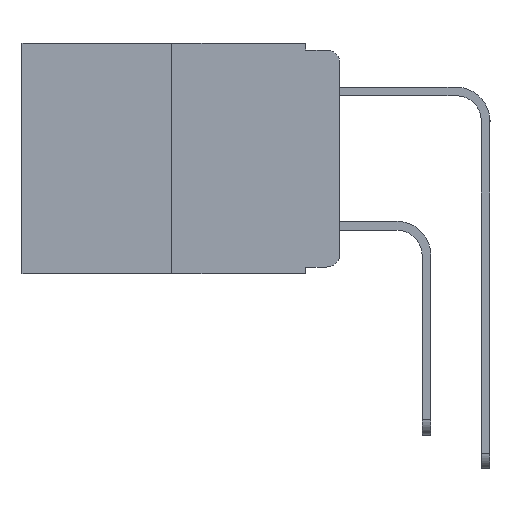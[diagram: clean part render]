
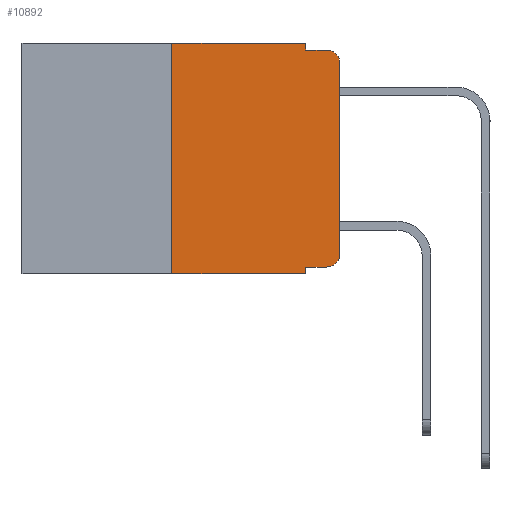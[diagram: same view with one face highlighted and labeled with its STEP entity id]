
A CAD part, left-side view. The second image highlights one B-rep face of the part: STEP entity #10892.
In plain terms, the highlighted planar face has unit normal (-1, 0, 0).
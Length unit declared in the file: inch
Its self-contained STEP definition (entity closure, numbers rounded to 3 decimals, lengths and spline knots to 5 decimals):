
#86 = VERTEX_POINT ( 'NONE', #1285 ) ;
#115 = CARTESIAN_POINT ( 'NONE',  ( 0., 0.051, -0.333 ) ) ;
#425 = VECTOR ( 'NONE', #3945, 39.37008 ) ;
#509 = VERTEX_POINT ( 'NONE', #13855 ) ;
#835 = CARTESIAN_POINT ( 'NONE',  ( 0., 0.02, -0.03 ) ) ;
#933 = LINE ( 'NONE', #15939, #8012 ) ;
#1285 = CARTESIAN_POINT ( 'NONE',  ( 0., 0.051, 0. ) ) ;
#1426 = VECTOR ( 'NONE', #2338, 39.37008 ) ;
#1512 = VERTEX_POINT ( 'NONE', #11597 ) ;
#2338 = DIRECTION ( 'NONE',  ( 0., 0., 1. ) ) ;
#2405 = DIRECTION ( 'NONE',  ( 0., 0., -1. ) ) ;
#2506 = PLANE ( 'NONE',  #4521 ) ;
#2543 = DIRECTION ( 'NONE',  ( -1., 0., 0. ) ) ;
#2708 = CARTESIAN_POINT ( 'NONE',  ( 0., 0., -0.03 ) ) ;
#2984 = AXIS2_PLACEMENT_3D ( 'NONE', #835, #10564, #2405 ) ;
#3136 = VERTEX_POINT ( 'NONE', #115 ) ;
#3711 = VERTEX_POINT ( 'NONE', #16877 ) ;
#3806 = ORIENTED_EDGE ( 'NONE', *, *, #12491, .F. ) ;
#3874 = DIRECTION ( 'NONE',  ( 0., 0., -1. ) ) ;
#3945 = DIRECTION ( 'NONE',  ( 0., -1., 0. ) ) ;
#4009 = CIRCLE ( 'NONE', #4880, 0.02 ) ;
#4450 = LINE ( 'NONE', #14625, #425 ) ;
#4521 = AXIS2_PLACEMENT_3D ( 'NONE', #15959, #8034, #17279 ) ;
#4576 = ORIENTED_EDGE ( 'NONE', *, *, #12466, .T. ) ;
#4861 = LINE ( 'NONE', #15879, #15530 ) ;
#4880 = AXIS2_PLACEMENT_3D ( 'NONE', #10687, #2543, #12038 ) ;
#5078 = ORIENTED_EDGE ( 'NONE', *, *, #12472, .F. ) ;
#5169 = DIRECTION ( 'NONE',  ( 0., -1., 0. ) ) ;
#6206 = ORIENTED_EDGE ( 'NONE', *, *, #12239, .T. ) ;
#6350 = ORIENTED_EDGE ( 'NONE', *, *, #12498, .T. ) ;
#6614 = DIRECTION ( 'NONE',  ( 0., -1., 0. ) ) ;
#6674 = DIRECTION ( 'NONE',  ( 0., 0., 1. ) ) ;
#7125 = VERTEX_POINT ( 'NONE', #2708 ) ;
#7220 = CARTESIAN_POINT ( 'NONE',  ( 0., 0.25, 0. ) ) ;
#7296 = ORIENTED_EDGE ( 'NONE', *, *, #12518, .T. ) ;
#7422 = DIRECTION ( 'NONE',  ( 0., -1., 0. ) ) ;
#8012 = VECTOR ( 'NONE', #6674, 39.37008 ) ;
#8034 = DIRECTION ( 'NONE',  ( 1., 0., 0. ) ) ;
#8382 = CIRCLE ( 'NONE', #2984, 0.02 ) ;
#8410 = VERTEX_POINT ( 'NONE', #8828 ) ;
#8828 = CARTESIAN_POINT ( 'NONE',  ( 0., 0.02, -0.333 ) ) ;
#9134 = CARTESIAN_POINT ( 'NONE',  ( 0., 0., 0. ) ) ;
#9140 = LINE ( 'NONE', #13176, #10414 ) ;
#9146 = VERTEX_POINT ( 'NONE', #7220 ) ;
#9201 = CARTESIAN_POINT ( 'NONE',  ( 0., 0.051, 0. ) ) ;
#9471 = ORIENTED_EDGE ( 'NONE', *, *, #12452, .T. ) ;
#10164 = VERTEX_POINT ( 'NONE', #14168 ) ;
#10378 = CARTESIAN_POINT ( 'NONE',  ( 0., 0.02, -0.01 ) ) ;
#10414 = VECTOR ( 'NONE', #5169, 39.37008 ) ;
#10564 = DIRECTION ( 'NONE',  ( -1., 0., 0. ) ) ;
#10623 = DIRECTION ( 'NONE',  ( 0., 0., -1. ) ) ;
#10687 = CARTESIAN_POINT ( 'NONE',  ( 0., 0.02, -0.313 ) ) ;
#10750 = ORIENTED_EDGE ( 'NONE', *, *, #12494, .F. ) ;
#10892 = ADVANCED_FACE ( 'NONE', ( #11276 ), #2506, .F. ) ;
#11276 = FACE_OUTER_BOUND ( 'NONE', #14150, .T. ) ;
#11597 = CARTESIAN_POINT ( 'NONE',  ( 0., 0.051, -0.343 ) ) ;
#11916 = EDGE_CURVE ( 'NONE', #9146, #86, #9140, .T. ) ;
#11980 = LINE ( 'NONE', #9201, #15124 ) ;
#12038 = DIRECTION ( 'NONE',  ( 0., 0., -1. ) ) ;
#12239 = EDGE_CURVE ( 'NONE', #509, #1512, #16920, .T. ) ;
#12418 = LINE ( 'NONE', #9134, #1426 ) ;
#12452 = EDGE_CURVE ( 'NONE', #3711, #7125, #12418, .T. ) ;
#12466 = EDGE_CURVE ( 'NONE', #7125, #17675, #8382, .T. ) ;
#12469 = EDGE_CURVE ( 'NONE', #10164, #17675, #4861, .T. ) ;
#12472 = EDGE_CURVE ( 'NONE', #86, #10164, #11980, .T. ) ;
#12491 = EDGE_CURVE ( 'NONE', #509, #9146, #933, .T. ) ;
#12494 = EDGE_CURVE ( 'NONE', #3136, #1512, #15937, .T. ) ;
#12498 = EDGE_CURVE ( 'NONE', #3136, #8410, #4450, .T. ) ;
#12518 = EDGE_CURVE ( 'NONE', #8410, #3711, #4009, .T. ) ;
#13176 = CARTESIAN_POINT ( 'NONE',  ( 0., 0.473, 0. ) ) ;
#13490 = ORIENTED_EDGE ( 'NONE', *, *, #11916, .F. ) ;
#13855 = CARTESIAN_POINT ( 'NONE',  ( 0., 0.25, -0.343 ) ) ;
#14071 = CARTESIAN_POINT ( 'NONE',  ( 0., 0.473, -0.343 ) ) ;
#14150 = EDGE_LOOP ( 'NONE', ( #9471, #4576, #15252, #5078, #13490, #3806, #6206, #10750, #6350, #7296 ) ) ;
#14168 = CARTESIAN_POINT ( 'NONE',  ( 0., 0.051, -0.01 ) ) ;
#14625 = CARTESIAN_POINT ( 'NONE',  ( 0., 0.051, -0.333 ) ) ;
#14713 = VECTOR ( 'NONE', #10623, 39.37008 ) ;
#15124 = VECTOR ( 'NONE', #3874, 39.37008 ) ;
#15252 = ORIENTED_EDGE ( 'NONE', *, *, #12469, .F. ) ;
#15530 = VECTOR ( 'NONE', #6614, 39.37008 ) ;
#15879 = CARTESIAN_POINT ( 'NONE',  ( 0., 0.051, -0.01 ) ) ;
#15937 = LINE ( 'NONE', #17199, #14713 ) ;
#15939 = CARTESIAN_POINT ( 'NONE',  ( 0., 0.25, 0. ) ) ;
#15959 = CARTESIAN_POINT ( 'NONE',  ( 0., 0.473, 0. ) ) ;
#16523 = VECTOR ( 'NONE', #7422, 39.37008 ) ;
#16877 = CARTESIAN_POINT ( 'NONE',  ( 0., 0., -0.313 ) ) ;
#16920 = LINE ( 'NONE', #14071, #16523 ) ;
#17199 = CARTESIAN_POINT ( 'NONE',  ( 0., 0.051, 0. ) ) ;
#17279 = DIRECTION ( 'NONE',  ( 0., 0., -1. ) ) ;
#17675 = VERTEX_POINT ( 'NONE', #10378 ) ;
